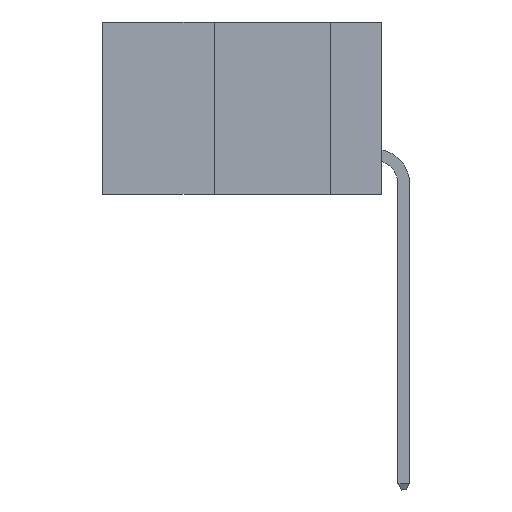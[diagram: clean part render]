
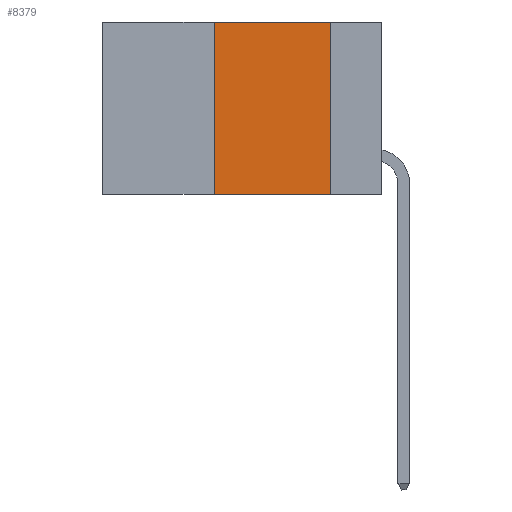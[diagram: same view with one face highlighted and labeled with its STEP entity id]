
A CAD part, left-side view. The second image highlights one B-rep face of the part: STEP entity #8379.
In plain terms, the highlighted planar face has unit normal (-1, 0, 0).
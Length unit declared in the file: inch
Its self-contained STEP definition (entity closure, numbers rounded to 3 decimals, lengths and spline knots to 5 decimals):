
#142 = VERTEX_POINT ( 'NONE', #3545 ) ;
#392 = VECTOR ( 'NONE', #3507, 39.37008 ) ;
#900 = DIRECTION ( 'NONE',  ( 0., -1., 0. ) ) ;
#1166 = EDGE_CURVE ( 'NONE', #11173, #6814, #9352, .T. ) ;
#1310 = CARTESIAN_POINT ( 'NONE',  ( 0., 0.6, 0. ) ) ;
#1725 = CARTESIAN_POINT ( 'NONE',  ( 0., 0.6, -0.37 ) ) ;
#2220 = VECTOR ( 'NONE', #10870, 39.37008 ) ;
#2635 = EDGE_CURVE ( 'NONE', #142, #5568, #4993, .T. ) ;
#2836 = LINE ( 'NONE', #1725, #392 ) ;
#3507 = DIRECTION ( 'NONE',  ( 0., -1., 0. ) ) ;
#3545 = CARTESIAN_POINT ( 'NONE',  ( 0., 0.11, 0. ) ) ;
#4004 = DIRECTION ( 'NONE',  ( 0., 0., -1. ) ) ;
#4299 = ORIENTED_EDGE ( 'NONE', *, *, #1166, .F. ) ;
#4712 = VECTOR ( 'NONE', #10811, 39.37008 ) ;
#4993 = LINE ( 'NONE', #5645, #4712 ) ;
#5279 = FACE_OUTER_BOUND ( 'NONE', #11261, .T. ) ;
#5568 = VERTEX_POINT ( 'NONE', #9302 ) ;
#5645 = CARTESIAN_POINT ( 'NONE',  ( 0., 0.11, 0. ) ) ;
#5745 = ORIENTED_EDGE ( 'NONE', *, *, #11278, .T. ) ;
#5780 = PLANE ( 'NONE',  #7475 ) ;
#6120 = ORIENTED_EDGE ( 'NONE', *, *, #2635, .F. ) ;
#6814 = VERTEX_POINT ( 'NONE', #8952 ) ;
#7475 = AXIS2_PLACEMENT_3D ( 'NONE', #1310, #9371, #4004 ) ;
#7559 = ORIENTED_EDGE ( 'NONE', *, *, #8094, .F. ) ;
#8094 = EDGE_CURVE ( 'NONE', #6814, #142, #10604, .T. ) ;
#8379 = ADVANCED_FACE ( 'NONE', ( #5279 ), #5780, .F. ) ;
#8952 = CARTESIAN_POINT ( 'NONE',  ( 0., 0.36, 0. ) ) ;
#9302 = CARTESIAN_POINT ( 'NONE',  ( 0., 0.11, -0.37 ) ) ;
#9352 = LINE ( 'NONE', #10762, #2220 ) ;
#9371 = DIRECTION ( 'NONE',  ( 1., 0., 0. ) ) ;
#10350 = VECTOR ( 'NONE', #900, 39.37008 ) ;
#10374 = CARTESIAN_POINT ( 'NONE',  ( 0., 0.36, -0.37 ) ) ;
#10604 = LINE ( 'NONE', #11419, #10350 ) ;
#10762 = CARTESIAN_POINT ( 'NONE',  ( 0., 0.36, 0. ) ) ;
#10811 = DIRECTION ( 'NONE',  ( 0., 0., -1. ) ) ;
#10870 = DIRECTION ( 'NONE',  ( 0., 0., 1. ) ) ;
#11173 = VERTEX_POINT ( 'NONE', #10374 ) ;
#11261 = EDGE_LOOP ( 'NONE', ( #6120, #7559, #4299, #5745 ) ) ;
#11278 = EDGE_CURVE ( 'NONE', #11173, #5568, #2836, .T. ) ;
#11419 = CARTESIAN_POINT ( 'NONE',  ( 0., 0.6, 0. ) ) ;
